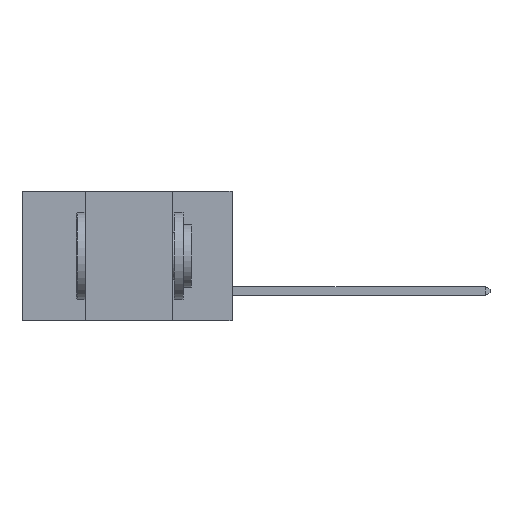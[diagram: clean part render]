
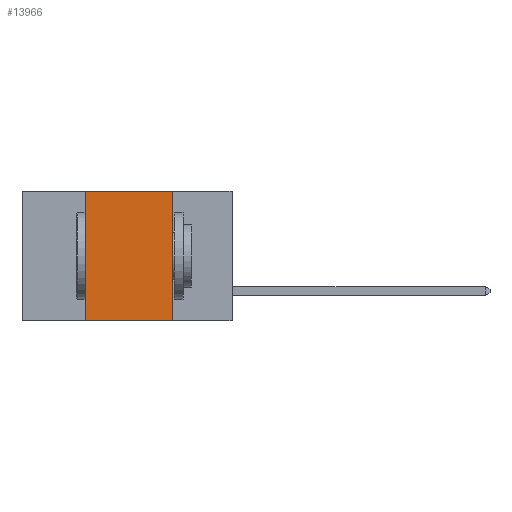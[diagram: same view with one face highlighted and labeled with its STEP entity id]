
A CAD part, left-side view. The second image highlights one B-rep face of the part: STEP entity #13966.
In plain terms, the highlighted planar face has unit normal (-1, 0, 0).
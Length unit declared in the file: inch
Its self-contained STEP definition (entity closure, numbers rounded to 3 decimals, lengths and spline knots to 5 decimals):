
#871 = VERTEX_POINT ( 'NONE', #24416 ) ;
#1064 = VERTEX_POINT ( 'NONE', #19339 ) ;
#1740 = VERTEX_POINT ( 'NONE', #6628 ) ;
#2478 = VECTOR ( 'NONE', #22294, 39.37008 ) ;
#2900 = CARTESIAN_POINT ( 'NONE',  ( 0., 0.42, 0. ) ) ;
#3417 = ORIENTED_EDGE ( 'NONE', *, *, #4632, .T. ) ;
#3778 = VECTOR ( 'NONE', #24109, 39.37008 ) ;
#4461 = LINE ( 'NONE', #20001, #3778 ) ;
#4632 = EDGE_CURVE ( 'NONE', #871, #22532, #19225, .T. ) ;
#6628 = CARTESIAN_POINT ( 'NONE',  ( 0., 0.42, 0. ) ) ;
#7046 = DIRECTION ( 'NONE',  ( 0., 0., -1. ) ) ;
#7142 = VECTOR ( 'NONE', #7046, 39.37008 ) ;
#7725 = EDGE_CURVE ( 'NONE', #1740, #1064, #4461, .T. ) ;
#8449 = LINE ( 'NONE', #2900, #2478 ) ;
#9022 = FACE_OUTER_BOUND ( 'NONE', #12235, .T. ) ;
#10250 = EDGE_CURVE ( 'NONE', #1064, #22532, #12976, .T. ) ;
#12123 = ORIENTED_EDGE ( 'NONE', *, *, #10250, .F. ) ;
#12235 = EDGE_LOOP ( 'NONE', ( #12123, #13492, #14467, #3417 ) ) ;
#12624 = EDGE_CURVE ( 'NONE', #871, #1740, #8449, .T. ) ;
#12976 = LINE ( 'NONE', #13581, #7142 ) ;
#13021 = DIRECTION ( 'NONE',  ( 0., 0., -1. ) ) ;
#13045 = DIRECTION ( 'NONE',  ( 0., -1., 0. ) ) ;
#13492 = ORIENTED_EDGE ( 'NONE', *, *, #7725, .F. ) ;
#13581 = CARTESIAN_POINT ( 'NONE',  ( 0., 0.17, 0. ) ) ;
#13682 = VECTOR ( 'NONE', #13045, 39.37008 ) ;
#13966 = ADVANCED_FACE ( 'NONE', ( #9022 ), #23453, .F. ) ;
#14467 = ORIENTED_EDGE ( 'NONE', *, *, #12624, .F. ) ;
#15740 = CARTESIAN_POINT ( 'NONE',  ( 0., 0.17, -0.37 ) ) ;
#17837 = AXIS2_PLACEMENT_3D ( 'NONE', #21330, #25575, #13021 ) ;
#19225 = LINE ( 'NONE', #27658, #13682 ) ;
#19339 = CARTESIAN_POINT ( 'NONE',  ( 0., 0.17, 0. ) ) ;
#20001 = CARTESIAN_POINT ( 'NONE',  ( 0., 0.6, 0. ) ) ;
#21330 = CARTESIAN_POINT ( 'NONE',  ( 0., 0.6, 0. ) ) ;
#22294 = DIRECTION ( 'NONE',  ( 0., 0., 1. ) ) ;
#22532 = VERTEX_POINT ( 'NONE', #15740 ) ;
#23453 = PLANE ( 'NONE',  #17837 ) ;
#24109 = DIRECTION ( 'NONE',  ( 0., -1., 0. ) ) ;
#24416 = CARTESIAN_POINT ( 'NONE',  ( 0., 0.42, -0.37 ) ) ;
#25575 = DIRECTION ( 'NONE',  ( 1., 0., 0. ) ) ;
#27658 = CARTESIAN_POINT ( 'NONE',  ( 0., 0.6, -0.37 ) ) ;
